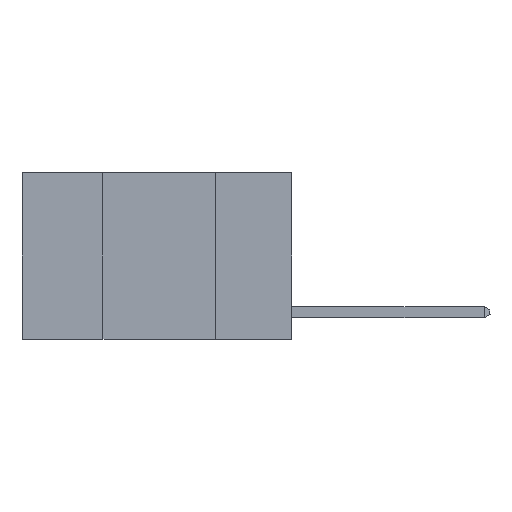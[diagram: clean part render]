
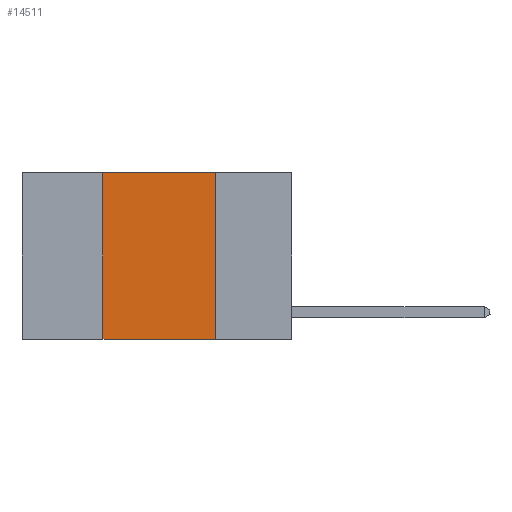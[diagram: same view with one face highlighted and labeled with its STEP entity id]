
A CAD part, left-side view. The second image highlights one B-rep face of the part: STEP entity #14511.
In plain terms, the highlighted planar face has unit normal (-1, 0, 0).
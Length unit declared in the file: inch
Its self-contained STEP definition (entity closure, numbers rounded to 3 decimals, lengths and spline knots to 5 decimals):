
#35 = CARTESIAN_POINT ( 'NONE',  ( 0., 0.17, -0.37 ) ) ;
#985 = CARTESIAN_POINT ( 'NONE',  ( 0., 0.6, 0. ) ) ;
#1337 = ORIENTED_EDGE ( 'NONE', *, *, #19735, .F. ) ;
#2657 = VECTOR ( 'NONE', #17028, 39.37008 ) ;
#3795 = CARTESIAN_POINT ( 'NONE',  ( 0., 0.17, 0. ) ) ;
#3970 = EDGE_CURVE ( 'NONE', #18179, #22795, #17254, .T. ) ;
#4352 = EDGE_LOOP ( 'NONE', ( #5377, #10194, #1337, #19287 ) ) ;
#5377 = ORIENTED_EDGE ( 'NONE', *, *, #5439, .F. ) ;
#5439 = EDGE_CURVE ( 'NONE', #22795, #9645, #7335, .T. ) ;
#7335 = LINE ( 'NONE', #3795, #18453 ) ;
#7477 = DIRECTION ( 'NONE',  ( 0., 0., -1. ) ) ;
#7601 = DIRECTION ( 'NONE',  ( 1., 0., 0. ) ) ;
#7908 = CARTESIAN_POINT ( 'NONE',  ( 0., 0.42, 0. ) ) ;
#7975 = CARTESIAN_POINT ( 'NONE',  ( 0., 0.42, -0.37 ) ) ;
#8385 = VECTOR ( 'NONE', #12525, 39.37008 ) ;
#9279 = FACE_OUTER_BOUND ( 'NONE', #4352, .T. ) ;
#9645 = VERTEX_POINT ( 'NONE', #35 ) ;
#10194 = ORIENTED_EDGE ( 'NONE', *, *, #3970, .F. ) ;
#10802 = DIRECTION ( 'NONE',  ( 0., 0., -1. ) ) ;
#11139 = EDGE_CURVE ( 'NONE', #14140, #9645, #22170, .T. ) ;
#12525 = DIRECTION ( 'NONE',  ( 0., -1., 0. ) ) ;
#12972 = PLANE ( 'NONE',  #20667 ) ;
#13884 = LINE ( 'NONE', #15796, #19061 ) ;
#14140 = VERTEX_POINT ( 'NONE', #7975 ) ;
#14511 = ADVANCED_FACE ( 'NONE', ( #9279 ), #12972, .F. ) ;
#15796 = CARTESIAN_POINT ( 'NONE',  ( 0., 0.42, 0. ) ) ;
#16120 = DIRECTION ( 'NONE',  ( 0., 0., 1. ) ) ;
#17028 = DIRECTION ( 'NONE',  ( 0., -1., 0. ) ) ;
#17254 = LINE ( 'NONE', #985, #8385 ) ;
#18179 = VERTEX_POINT ( 'NONE', #7908 ) ;
#18453 = VECTOR ( 'NONE', #10802, 39.37008 ) ;
#19061 = VECTOR ( 'NONE', #16120, 39.37008 ) ;
#19287 = ORIENTED_EDGE ( 'NONE', *, *, #11139, .T. ) ;
#19735 = EDGE_CURVE ( 'NONE', #14140, #18179, #13884, .T. ) ;
#19742 = CARTESIAN_POINT ( 'NONE',  ( 0., 0.17, 0. ) ) ;
#20242 = CARTESIAN_POINT ( 'NONE',  ( 0., 0.6, 0. ) ) ;
#20513 = CARTESIAN_POINT ( 'NONE',  ( 0., 0.6, -0.37 ) ) ;
#20667 = AXIS2_PLACEMENT_3D ( 'NONE', #20242, #7601, #7477 ) ;
#22170 = LINE ( 'NONE', #20513, #2657 ) ;
#22795 = VERTEX_POINT ( 'NONE', #19742 ) ;
